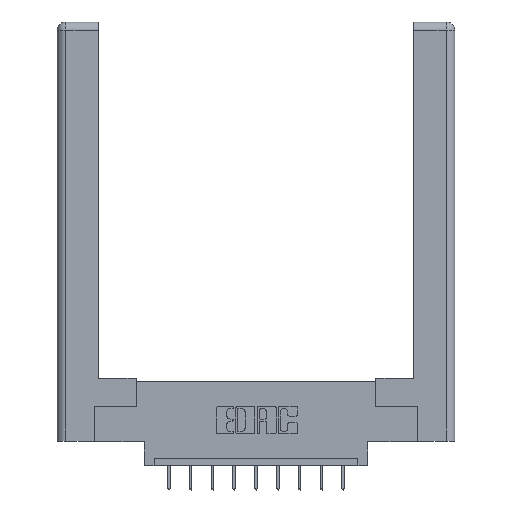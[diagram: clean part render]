
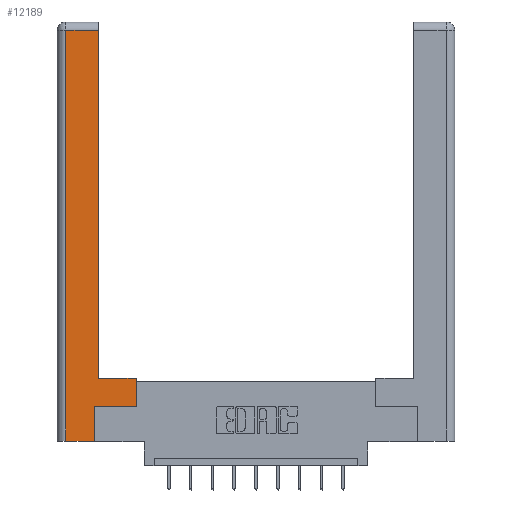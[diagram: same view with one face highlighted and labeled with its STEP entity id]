
A CAD part, top view. The second image highlights one B-rep face of the part: STEP entity #12189.
In plain terms, the highlighted planar face has unit normal (0, 0, 1).
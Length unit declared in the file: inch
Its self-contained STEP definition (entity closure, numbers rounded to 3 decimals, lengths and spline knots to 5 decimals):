
#200 = CARTESIAN_POINT ( 'NONE',  ( 0., 0., 0. ) ) ;
#552 = LINE ( 'NONE', #7030, #11578 ) ;
#652 = EDGE_CURVE ( 'NONE', #6587, #12169, #11693, .T. ) ;
#1174 = VECTOR ( 'NONE', #11105, 39.37008 ) ;
#1200 = VERTEX_POINT ( 'NONE', #8019 ) ;
#1619 = CARTESIAN_POINT ( 'NONE',  ( 0.295, 0.45, 0. ) ) ;
#1735 = CARTESIAN_POINT ( 'NONE',  ( 0.0615, 2.94, 0. ) ) ;
#1736 = EDGE_CURVE ( 'NONE', #2495, #1200, #9820, .T. ) ;
#2031 = ORIENTED_EDGE ( 'NONE', *, *, #10815, .T. ) ;
#2097 = CARTESIAN_POINT ( 'NONE',  ( 0.0615, 2.94, 0. ) ) ;
#2495 = VERTEX_POINT ( 'NONE', #5781 ) ;
#2841 = ORIENTED_EDGE ( 'NONE', *, *, #8979, .T. ) ;
#3171 = LINE ( 'NONE', #13745, #6527 ) ;
#3297 = PLANE ( 'NONE',  #12898 ) ;
#3319 = CARTESIAN_POINT ( 'NONE',  ( 0.295, 0.45, 0. ) ) ;
#3350 = CARTESIAN_POINT ( 'NONE',  ( 0.0615, 0., 0. ) ) ;
#3438 = DIRECTION ( 'NONE',  ( 0., -1., 0. ) ) ;
#4853 = VECTOR ( 'NONE', #3438, 39.37008 ) ;
#5182 = VECTOR ( 'NONE', #10023, 39.37008 ) ;
#5377 = CARTESIAN_POINT ( 'NONE',  ( 0.265, 0., 0. ) ) ;
#5482 = CARTESIAN_POINT ( 'NONE',  ( 0.565, 0.245, 0. ) ) ;
#5538 = DIRECTION ( 'NONE',  ( -1., 0., 0. ) ) ;
#5593 = LINE ( 'NONE', #3319, #8082 ) ;
#5781 = CARTESIAN_POINT ( 'NONE',  ( 0.265, 0., 0. ) ) ;
#5888 = VERTEX_POINT ( 'NONE', #1619 ) ;
#6174 = DIRECTION ( 'NONE',  ( 0., 1., 0. ) ) ;
#6320 = EDGE_CURVE ( 'NONE', #12169, #2495, #13276, .T. ) ;
#6435 = DIRECTION ( 'NONE',  ( 1., 0., 0. ) ) ;
#6527 = VECTOR ( 'NONE', #6174, 39.37008 ) ;
#6587 = VERTEX_POINT ( 'NONE', #2097 ) ;
#7030 = CARTESIAN_POINT ( 'NONE',  ( 0.565, 0.45, 0. ) ) ;
#7110 = ORIENTED_EDGE ( 'NONE', *, *, #652, .T. ) ;
#7463 = EDGE_CURVE ( 'NONE', #12269, #5888, #5593, .T. ) ;
#7906 = CARTESIAN_POINT ( 'NONE',  ( 0.0615, 0., 0. ) ) ;
#8019 = CARTESIAN_POINT ( 'NONE',  ( 0.265, 0.245, 0. ) ) ;
#8082 = VECTOR ( 'NONE', #11754, 39.37008 ) ;
#8169 = EDGE_LOOP ( 'NONE', ( #11082, #8943, #7110, #10341, #13739, #2841, #2031, #9791 ) ) ;
#8516 = VECTOR ( 'NONE', #13555, 39.37008 ) ;
#8943 = ORIENTED_EDGE ( 'NONE', *, *, #9941, .T. ) ;
#8979 = EDGE_CURVE ( 'NONE', #1200, #9765, #9864, .T. ) ;
#9513 = EDGE_CURVE ( 'NONE', #5888, #11948, #3171, .T. ) ;
#9599 = VECTOR ( 'NONE', #6435, 39.37008 ) ;
#9765 = VERTEX_POINT ( 'NONE', #11829 ) ;
#9791 = ORIENTED_EDGE ( 'NONE', *, *, #7463, .T. ) ;
#9820 = LINE ( 'NONE', #11958, #5182 ) ;
#9839 = FACE_OUTER_BOUND ( 'NONE', #8169, .T. ) ;
#9864 = LINE ( 'NONE', #5482, #1174 ) ;
#9941 = EDGE_CURVE ( 'NONE', #11948, #6587, #11700, .T. ) ;
#10023 = DIRECTION ( 'NONE',  ( 0., 1., 0. ) ) ;
#10341 = ORIENTED_EDGE ( 'NONE', *, *, #6320, .T. ) ;
#10478 = DIRECTION ( 'NONE',  ( 0., 1., 0. ) ) ;
#10815 = EDGE_CURVE ( 'NONE', #9765, #12269, #552, .T. ) ;
#11082 = ORIENTED_EDGE ( 'NONE', *, *, #9513, .T. ) ;
#11105 = DIRECTION ( 'NONE',  ( 1., 0., 0. ) ) ;
#11578 = VECTOR ( 'NONE', #10478, 39.37008 ) ;
#11693 = LINE ( 'NONE', #7906, #4853 ) ;
#11700 = LINE ( 'NONE', #1735, #8516 ) ;
#11754 = DIRECTION ( 'NONE',  ( -1., 0., 0. ) ) ;
#11829 = CARTESIAN_POINT ( 'NONE',  ( 0.565, 0.245, 0. ) ) ;
#11863 = DIRECTION ( 'NONE',  ( 0., 0., -1. ) ) ;
#11948 = VERTEX_POINT ( 'NONE', #12373 ) ;
#11958 = CARTESIAN_POINT ( 'NONE',  ( 0.265, 0.245, 0. ) ) ;
#12006 = CARTESIAN_POINT ( 'NONE',  ( 0.565, 0.45, 0. ) ) ;
#12169 = VERTEX_POINT ( 'NONE', #3350 ) ;
#12189 = ADVANCED_FACE ( 'NONE', ( #9839 ), #3297, .F. ) ;
#12269 = VERTEX_POINT ( 'NONE', #12006 ) ;
#12373 = CARTESIAN_POINT ( 'NONE',  ( 0.295, 2.94, 0. ) ) ;
#12898 = AXIS2_PLACEMENT_3D ( 'NONE', #200, #11863, #5538 ) ;
#13276 = LINE ( 'NONE', #5377, #9599 ) ;
#13555 = DIRECTION ( 'NONE',  ( -1., 0., 0. ) ) ;
#13739 = ORIENTED_EDGE ( 'NONE', *, *, #1736, .T. ) ;
#13745 = CARTESIAN_POINT ( 'NONE',  ( 0.295, 3., 0. ) ) ;
